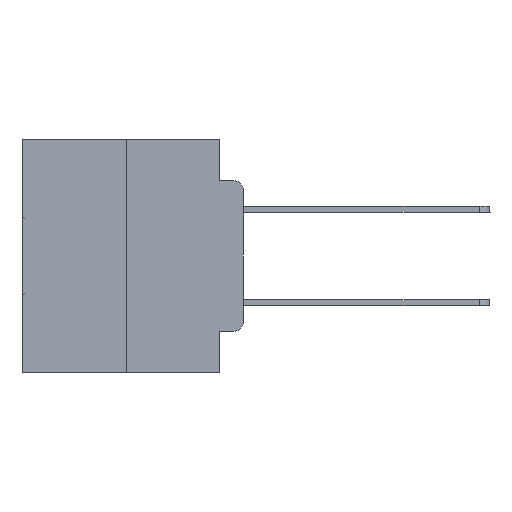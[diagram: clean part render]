
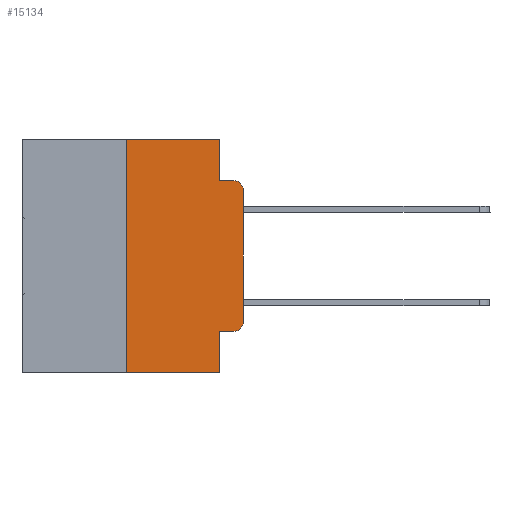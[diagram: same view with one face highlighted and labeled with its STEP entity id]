
A CAD part, left-side view. The second image highlights one B-rep face of the part: STEP entity #15134.
In plain terms, the highlighted planar face has unit normal (-1, 0, 0).
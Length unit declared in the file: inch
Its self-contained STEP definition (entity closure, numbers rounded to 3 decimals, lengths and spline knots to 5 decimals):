
#510 = LINE ( 'NONE', #21347, #22368 ) ;
#1562 = LINE ( 'NONE', #24157, #26419 ) ;
#1994 = EDGE_LOOP ( 'NONE', ( #25398, #5802, #15644, #7359, #3121, #10669, #25060, #17387, #23854, #27166 ) ) ;
#2156 = LINE ( 'NONE', #22782, #16878 ) ;
#2236 = PLANE ( 'NONE',  #21587 ) ;
#2448 = VECTOR ( 'NONE', #3175, 39.37008 ) ;
#2815 = VERTEX_POINT ( 'NONE', #4319 ) ;
#3121 = ORIENTED_EDGE ( 'NONE', *, *, #30325, .F. ) ;
#3175 = DIRECTION ( 'NONE',  ( 0., 0., 1. ) ) ;
#3940 = DIRECTION ( 'NONE',  ( 0., -1., 0. ) ) ;
#4083 = DIRECTION ( 'NONE',  ( 0., -1., 0. ) ) ;
#4297 = CARTESIAN_POINT ( 'NONE',  ( 0., 0.02, -0.0885 ) ) ;
#4319 = CARTESIAN_POINT ( 'NONE',  ( 0., 0.25, -0.5 ) ) ;
#4558 = DIRECTION ( 'NONE',  ( 0., 0., -1. ) ) ;
#4633 = VERTEX_POINT ( 'NONE', #10203 ) ;
#4881 = CARTESIAN_POINT ( 'NONE',  ( 0., 0.25, 0. ) ) ;
#5236 = VECTOR ( 'NONE', #30239, 39.37008 ) ;
#5802 = ORIENTED_EDGE ( 'NONE', *, *, #14424, .T. ) ;
#5914 = DIRECTION ( 'NONE',  ( -1., 0., 0. ) ) ;
#6137 = CARTESIAN_POINT ( 'NONE',  ( 0., 0.051, -0.0885 ) ) ;
#6764 = LINE ( 'NONE', #10415, #24439 ) ;
#7359 = ORIENTED_EDGE ( 'NONE', *, *, #13535, .F. ) ;
#7849 = DIRECTION ( 'NONE',  ( 0., 0., -1. ) ) ;
#8239 = CARTESIAN_POINT ( 'NONE',  ( 0., 0.25, 0. ) ) ;
#8903 = VERTEX_POINT ( 'NONE', #6137 ) ;
#9335 = CARTESIAN_POINT ( 'NONE',  ( 0., 0.051, 0. ) ) ;
#9568 = CARTESIAN_POINT ( 'NONE',  ( 0., 0.051, -0.0885 ) ) ;
#9773 = DIRECTION ( 'NONE',  ( 0., -1., 0. ) ) ;
#9813 = AXIS2_PLACEMENT_3D ( 'NONE', #29908, #19396, #7849 ) ;
#10203 = CARTESIAN_POINT ( 'NONE',  ( 0., 0., -0.1085 ) ) ;
#10415 = CARTESIAN_POINT ( 'NONE',  ( 0., 0.051, 0. ) ) ;
#10669 = ORIENTED_EDGE ( 'NONE', *, *, #21844, .F. ) ;
#11580 = FACE_OUTER_BOUND ( 'NONE', #1994, .T. ) ;
#11979 = EDGE_CURVE ( 'NONE', #26013, #22873, #1562, .T. ) ;
#12031 = LINE ( 'NONE', #22881, #5236 ) ;
#12677 = CARTESIAN_POINT ( 'NONE',  ( 0., 0., 0. ) ) ;
#12745 = VERTEX_POINT ( 'NONE', #23475 ) ;
#12897 = LINE ( 'NONE', #8239, #25669 ) ;
#13535 = EDGE_CURVE ( 'NONE', #19176, #8903, #6764, .T. ) ;
#13594 = EDGE_CURVE ( 'NONE', #26013, #30893, #12031, .T. ) ;
#14424 = EDGE_CURVE ( 'NONE', #4633, #25982, #18723, .T. ) ;
#15134 = ADVANCED_FACE ( 'NONE', ( #11580 ), #2236, .F. ) ;
#15619 = DIRECTION ( 'NONE',  ( 0., 0., -1. ) ) ;
#15644 = ORIENTED_EDGE ( 'NONE', *, *, #27938, .F. ) ;
#15667 = EDGE_CURVE ( 'NONE', #12745, #4633, #30676, .T. ) ;
#16878 = VECTOR ( 'NONE', #3940, 39.37008 ) ;
#17387 = ORIENTED_EDGE ( 'NONE', *, *, #13594, .F. ) ;
#18230 = VECTOR ( 'NONE', #28780, 39.37008 ) ;
#18723 = CIRCLE ( 'NONE', #23614, 0.02 ) ;
#18869 = EDGE_CURVE ( 'NONE', #2815, #30893, #2156, .T. ) ;
#19176 = VERTEX_POINT ( 'NONE', #9335 ) ;
#19330 = EDGE_CURVE ( 'NONE', #22873, #12745, #24735, .T. ) ;
#19396 = DIRECTION ( 'NONE',  ( -1., 0., 0. ) ) ;
#19957 = DIRECTION ( 'NONE',  ( 0., 0., -1. ) ) ;
#20233 = CARTESIAN_POINT ( 'NONE',  ( 0., 0.051, -0.5 ) ) ;
#20323 = CARTESIAN_POINT ( 'NONE',  ( 0., 0.02, -0.1085 ) ) ;
#21347 = CARTESIAN_POINT ( 'NONE',  ( 0., 0.473, 0. ) ) ;
#21587 = AXIS2_PLACEMENT_3D ( 'NONE', #26121, #26333, #4558 ) ;
#21844 = EDGE_CURVE ( 'NONE', #2815, #27883, #12897, .T. ) ;
#22368 = VECTOR ( 'NONE', #4083, 39.37008 ) ;
#22782 = CARTESIAN_POINT ( 'NONE',  ( 0., 0.473, -0.5 ) ) ;
#22873 = VERTEX_POINT ( 'NONE', #24348 ) ;
#22881 = CARTESIAN_POINT ( 'NONE',  ( 0., 0.051, 0. ) ) ;
#23475 = CARTESIAN_POINT ( 'NONE',  ( 0., 0., -0.3915 ) ) ;
#23614 = AXIS2_PLACEMENT_3D ( 'NONE', #20323, #5914, #15619 ) ;
#23767 = CARTESIAN_POINT ( 'NONE',  ( 0., 0.051, -0.4115 ) ) ;
#23854 = ORIENTED_EDGE ( 'NONE', *, *, #11979, .T. ) ;
#24157 = CARTESIAN_POINT ( 'NONE',  ( 0., 0.051, -0.4115 ) ) ;
#24348 = CARTESIAN_POINT ( 'NONE',  ( 0., 0.02, -0.4115 ) ) ;
#24439 = VECTOR ( 'NONE', #19957, 39.37008 ) ;
#24643 = LINE ( 'NONE', #9568, #18230 ) ;
#24735 = CIRCLE ( 'NONE', #9813, 0.02 ) ;
#25060 = ORIENTED_EDGE ( 'NONE', *, *, #18869, .T. ) ;
#25398 = ORIENTED_EDGE ( 'NONE', *, *, #15667, .T. ) ;
#25669 = VECTOR ( 'NONE', #27435, 39.37008 ) ;
#25982 = VERTEX_POINT ( 'NONE', #4297 ) ;
#26013 = VERTEX_POINT ( 'NONE', #23767 ) ;
#26121 = CARTESIAN_POINT ( 'NONE',  ( 0., 0.473, 0. ) ) ;
#26333 = DIRECTION ( 'NONE',  ( 1., 0., 0. ) ) ;
#26419 = VECTOR ( 'NONE', #9773, 39.37008 ) ;
#27166 = ORIENTED_EDGE ( 'NONE', *, *, #19330, .T. ) ;
#27435 = DIRECTION ( 'NONE',  ( 0., 0., 1. ) ) ;
#27883 = VERTEX_POINT ( 'NONE', #4881 ) ;
#27938 = EDGE_CURVE ( 'NONE', #8903, #25982, #24643, .T. ) ;
#28780 = DIRECTION ( 'NONE',  ( 0., -1., 0. ) ) ;
#29908 = CARTESIAN_POINT ( 'NONE',  ( 0., 0.02, -0.3915 ) ) ;
#30239 = DIRECTION ( 'NONE',  ( 0., 0., -1. ) ) ;
#30325 = EDGE_CURVE ( 'NONE', #27883, #19176, #510, .T. ) ;
#30676 = LINE ( 'NONE', #12677, #2448 ) ;
#30893 = VERTEX_POINT ( 'NONE', #20233 ) ;
